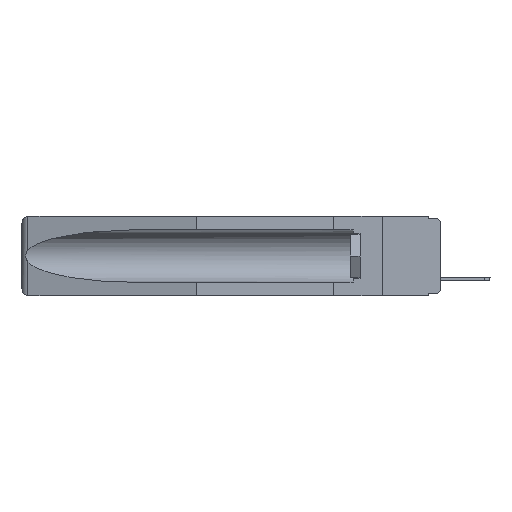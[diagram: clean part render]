
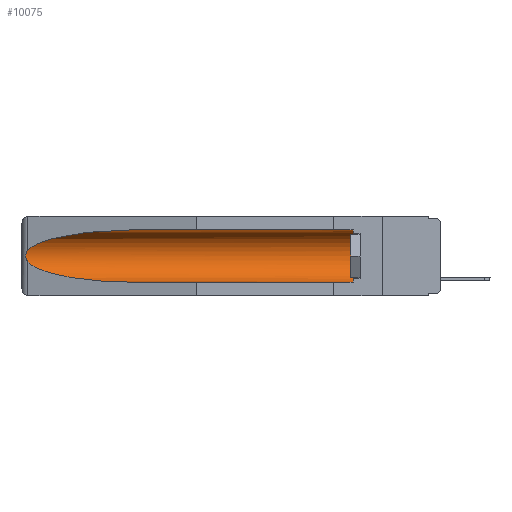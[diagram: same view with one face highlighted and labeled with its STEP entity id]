
A CAD part, left-side view. The second image highlights one B-rep face of the part: STEP entity #10075.
In plain terms, the highlighted cylindrical face has radius 2.857 mm (diameter 5.715 mm), a partial arc.
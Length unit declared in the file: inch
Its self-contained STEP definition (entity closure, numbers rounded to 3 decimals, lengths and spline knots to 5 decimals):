
#131 = VERTEX_POINT ( 'NONE', #6353 ) ;
#758 = EDGE_CURVE ( 'NONE', #19414, #7798, #12437, .T. ) ;
#1805 = ORIENTED_EDGE ( 'NONE', *, *, #19826, .T. ) ;
#1811 = CARTESIAN_POINT ( 'NONE',  ( 0.2675, 1.53308, -0.17534 ) ) ;
#1920 = ORIENTED_EDGE ( 'NONE', *, *, #13573, .F. ) ;
#2218 = EDGE_CURVE ( 'NONE', #131, #7735, #18707, .T. ) ;
#2510 = DIRECTION ( 'NONE',  ( 0., 1., 0. ) ) ;
#2932 = CARTESIAN_POINT ( 'NONE',  ( 0.21114, 1.30732, -0.059 ) ) ;
#3847 = CARTESIAN_POINT ( 'NONE',  ( 0.26654, 1.53092, -0.15636 ) ) ;
#3959 = VECTOR ( 'NONE', #10023, 39.37008 ) ;
#3966 = CARTESIAN_POINT ( 'NONE',  ( 0.26655, 1.53094, -0.18657 ) ) ;
#4385 = CARTESIAN_POINT ( 'NONE',  ( 0.155, -0.30754, -0.059 ) ) ;
#4780 = DIRECTION ( 'NONE',  ( 0., 0., 1. ) ) ;
#5479 = CARTESIAN_POINT ( 'NONE',  ( 0.25451, 1.48313, -0.09465 ) ) ;
#5752 = ORIENTED_EDGE ( 'NONE', *, *, #758, .T. ) ;
#5807 = ORIENTED_EDGE ( 'NONE', *, *, #2218, .T. ) ;
#6113 = CARTESIAN_POINT ( 'NONE',  ( 0.155, -0.30754, -0.284 ) ) ;
#6353 = CARTESIAN_POINT ( 'NONE',  ( 0.155, 0.126, -0.059 ) ) ;
#7493 = CARTESIAN_POINT ( 'NONE',  ( 0.26537, 1.52718, -0.14972 ) ) ;
#7735 = VERTEX_POINT ( 'NONE', #15464 ) ;
#7741 = CARTESIAN_POINT ( 'NONE',  ( 0.26597, 1.5296, -0.19026 ) ) ;
#7798 = VERTEX_POINT ( 'NONE', #19612 ) ;
#8011 = CARTESIAN_POINT ( 'NONE',  ( 0.26537, 1.52718, -0.19328 ) ) ;
#8160 = CARTESIAN_POINT ( 'NONE',  ( 0.26537, 1.52718, -0.14972 ) ) ;
#8603 = EDGE_CURVE ( 'NONE', #7735, #20161, #22599, .T. ) ;
#9383 = DIRECTION ( 'NONE',  ( 0., 0., 1. ) ) ;
#9771 = CARTESIAN_POINT ( 'NONE',  ( 0.26597, 1.52961, -0.15275 ) ) ;
#10023 = DIRECTION ( 'NONE',  ( 0., 1., 0. ) ) ;
#10075 = ADVANCED_FACE ( 'NONE', ( #22423 ), #16940, .F. ) ;
#10399 = EDGE_CURVE ( 'NONE', #20161, #19414, #25306, .T. ) ;
#11065 = AXIS2_PLACEMENT_3D ( 'NONE', #13030, #13562, #9383 ) ;
#12437 =( BOUNDED_CURVE ( )  B_SPLINE_CURVE ( 3, ( #24415, #13986, #18064, #19937 ),
 .UNSPECIFIED., .F., .F. ) 
 B_SPLINE_CURVE_WITH_KNOTS ( ( 4, 4 ),
 ( 0.1948, 1.5708 ),
 .UNSPECIFIED. ) 
 CURVE ( )  GEOMETRIC_REPRESENTATION_ITEM ( )  RATIONAL_B_SPLINE_CURVE ( ( 1., 0.848, 0.848, 1. ) ) 
 REPRESENTATION_ITEM ( '' )  );
#13030 = CARTESIAN_POINT ( 'NONE',  ( 0.155, 0.126, -0.1715 ) ) ;
#13562 = DIRECTION ( 'NONE',  ( 0., -1., 0. ) ) ;
#13573 = EDGE_CURVE ( 'NONE', #20852, #7798, #22478, .T. ) ;
#13986 = CARTESIAN_POINT ( 'NONE',  ( 0.25451, 1.48313, -0.24835 ) ) ;
#14105 = CARTESIAN_POINT ( 'NONE',  ( 0.2675, 1.53308, -0.16763 ) ) ;
#14557 = AXIS2_PLACEMENT_3D ( 'NONE', #23308, #24454, #4780 ) ;
#14664 = EDGE_LOOP ( 'NONE', ( #17563, #16017, #5752, #1920, #1805, #5807 ) ) ;
#15464 = CARTESIAN_POINT ( 'NONE',  ( 0.155, 1.07973, -0.059 ) ) ;
#15620 = CARTESIAN_POINT ( 'NONE',  ( 0.155, 1.07973, -0.059 ) ) ;
#15802 = CARTESIAN_POINT ( 'NONE',  ( 0.26537, 1.52718, -0.14972 ) ) ;
#16017 = ORIENTED_EDGE ( 'NONE', *, *, #10399, .T. ) ;
#16940 = CYLINDRICAL_SURFACE ( 'NONE', #14557, 0.1125 ) ;
#17563 = ORIENTED_EDGE ( 'NONE', *, *, #8603, .T. ) ;
#18064 = CARTESIAN_POINT ( 'NONE',  ( 0.21114, 1.30732, -0.284 ) ) ;
#18707 = LINE ( 'NONE', #4385, #20734 ) ;
#19414 = VERTEX_POINT ( 'NONE', #23471 ) ;
#19612 = CARTESIAN_POINT ( 'NONE',  ( 0.155, 1.07973, -0.284 ) ) ;
#19697 = CIRCLE ( 'NONE', #11065, 0.1125 ) ;
#19826 = EDGE_CURVE ( 'NONE', #20852, #131, #19697, .T. ) ;
#19937 = CARTESIAN_POINT ( 'NONE',  ( 0.155, 1.07973, -0.284 ) ) ;
#20161 = VERTEX_POINT ( 'NONE', #15802 ) ;
#20187 = CARTESIAN_POINT ( 'NONE',  ( 0.2673, 1.53269, -0.17917 ) ) ;
#20734 = VECTOR ( 'NONE', #2510, 39.37008 ) ;
#20852 = VERTEX_POINT ( 'NONE', #21263 ) ;
#21263 = CARTESIAN_POINT ( 'NONE',  ( 0.155, 0.126, -0.284 ) ) ;
#22423 = FACE_OUTER_BOUND ( 'NONE', #14664, .T. ) ;
#22478 = LINE ( 'NONE', #6113, #3959 ) ;
#22599 =( BOUNDED_CURVE ( )  B_SPLINE_CURVE ( 3, ( #15620, #2932, #5479, #7493 ),
 .UNSPECIFIED., .F., .F. ) 
 B_SPLINE_CURVE_WITH_KNOTS ( ( 4, 4 ),
 ( 4.71239, 6.08839 ),
 .UNSPECIFIED. ) 
 CURVE ( )  GEOMETRIC_REPRESENTATION_ITEM ( )  RATIONAL_B_SPLINE_CURVE ( ( 1., 0.848, 0.848, 1. ) ) 
 REPRESENTATION_ITEM ( '' )  );
#23308 = CARTESIAN_POINT ( 'NONE',  ( 0.155, -0.30754, -0.1715 ) ) ;
#23471 = CARTESIAN_POINT ( 'NONE',  ( 0.26537, 1.52718, -0.19328 ) ) ;
#24127 = CARTESIAN_POINT ( 'NONE',  ( 0.2673, 1.5327, -0.16383 ) ) ;
#24415 = CARTESIAN_POINT ( 'NONE',  ( 0.26537, 1.52718, -0.19328 ) ) ;
#24454 = DIRECTION ( 'NONE',  ( 0., 1., 0. ) ) ;
#25306 = B_SPLINE_CURVE_WITH_KNOTS ( 'NONE', 3,
 ( #8160, #9771, #3847, #24127, #14105, #1811, #20187, #3966, #7741, #8011 ),
 .UNSPECIFIED., .F., .F.,
 ( 4, 2, 2, 2, 4 ),
 ( 0., 0.00029, 0.00058, 0.00087, 0.00117 ),
 .UNSPECIFIED. ) ;
